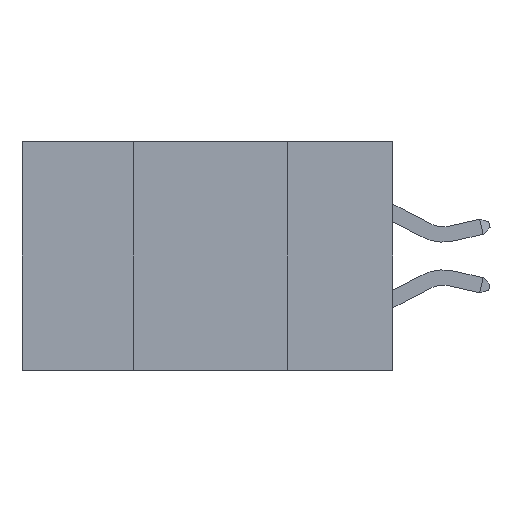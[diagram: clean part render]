
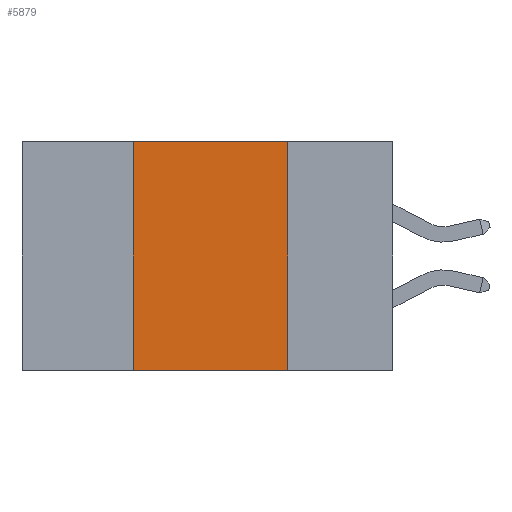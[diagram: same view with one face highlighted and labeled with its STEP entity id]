
A CAD part, left-side view. The second image highlights one B-rep face of the part: STEP entity #5879.
In plain terms, the highlighted planar face has unit normal (-1, 0, 0).
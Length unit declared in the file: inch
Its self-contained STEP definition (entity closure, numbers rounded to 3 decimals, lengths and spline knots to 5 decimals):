
#194 = CARTESIAN_POINT ( 'NONE',  ( 0., 0.6, 0. ) ) ;
#1439 = ORIENTED_EDGE ( 'NONE', *, *, #7444, .T. ) ;
#1453 = VECTOR ( 'NONE', #4889, 39.37008 ) ;
#2339 = DIRECTION ( 'NONE',  ( 0., -1., 0. ) ) ;
#2531 = VERTEX_POINT ( 'NONE', #12324 ) ;
#2604 = EDGE_CURVE ( 'NONE', #2822, #8571, #12155, .T. ) ;
#2822 = VERTEX_POINT ( 'NONE', #9153 ) ;
#3874 = CARTESIAN_POINT ( 'NONE',  ( 0., 0.42, 0. ) ) ;
#4165 = EDGE_CURVE ( 'NONE', #8571, #10668, #4201, .T. ) ;
#4201 = LINE ( 'NONE', #9049, #6916 ) ;
#4591 = ORIENTED_EDGE ( 'NONE', *, *, #4165, .F. ) ;
#4782 = DIRECTION ( 'NONE',  ( 0., 0., 1. ) ) ;
#4889 = DIRECTION ( 'NONE',  ( 0., 0., -1. ) ) ;
#4926 = CARTESIAN_POINT ( 'NONE',  ( 0., 0.17, 0. ) ) ;
#5643 = DIRECTION ( 'NONE',  ( 0., -1., 0. ) ) ;
#5854 = DIRECTION ( 'NONE',  ( 1., 0., 0. ) ) ;
#5879 = ADVANCED_FACE ( 'NONE', ( #9120 ), #11784, .F. ) ;
#6540 = LINE ( 'NONE', #8403, #11921 ) ;
#6916 = VECTOR ( 'NONE', #2339, 39.37008 ) ;
#7444 = EDGE_CURVE ( 'NONE', #2822, #2531, #6540, .T. ) ;
#7906 = DIRECTION ( 'NONE',  ( 0., 0., -1. ) ) ;
#8357 = LINE ( 'NONE', #4926, #1453 ) ;
#8403 = CARTESIAN_POINT ( 'NONE',  ( 0., 0.6, -0.37 ) ) ;
#8571 = VERTEX_POINT ( 'NONE', #9045 ) ;
#9045 = CARTESIAN_POINT ( 'NONE',  ( 0., 0.42, 0. ) ) ;
#9049 = CARTESIAN_POINT ( 'NONE',  ( 0., 0.6, 0. ) ) ;
#9120 = FACE_OUTER_BOUND ( 'NONE', #11852, .T. ) ;
#9153 = CARTESIAN_POINT ( 'NONE',  ( 0., 0.42, -0.37 ) ) ;
#9501 = ORIENTED_EDGE ( 'NONE', *, *, #11239, .F. ) ;
#10668 = VERTEX_POINT ( 'NONE', #11862 ) ;
#10845 = ORIENTED_EDGE ( 'NONE', *, *, #2604, .F. ) ;
#11239 = EDGE_CURVE ( 'NONE', #10668, #2531, #8357, .T. ) ;
#11283 = VECTOR ( 'NONE', #4782, 39.37008 ) ;
#11784 = PLANE ( 'NONE',  #11840 ) ;
#11840 = AXIS2_PLACEMENT_3D ( 'NONE', #194, #5854, #7906 ) ;
#11852 = EDGE_LOOP ( 'NONE', ( #9501, #4591, #10845, #1439 ) ) ;
#11862 = CARTESIAN_POINT ( 'NONE',  ( 0., 0.17, 0. ) ) ;
#11921 = VECTOR ( 'NONE', #5643, 39.37008 ) ;
#12155 = LINE ( 'NONE', #3874, #11283 ) ;
#12324 = CARTESIAN_POINT ( 'NONE',  ( 0., 0.17, -0.37 ) ) ;
